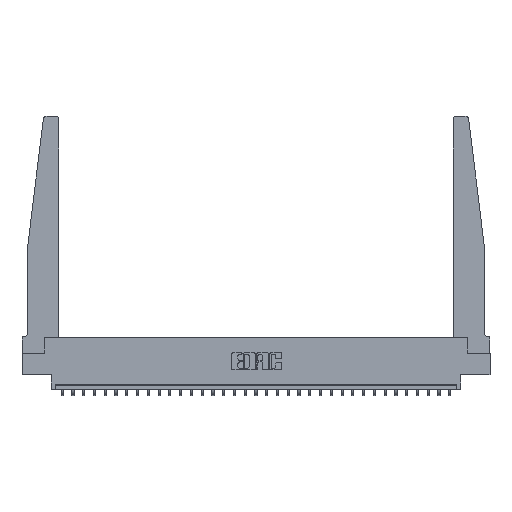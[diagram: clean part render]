
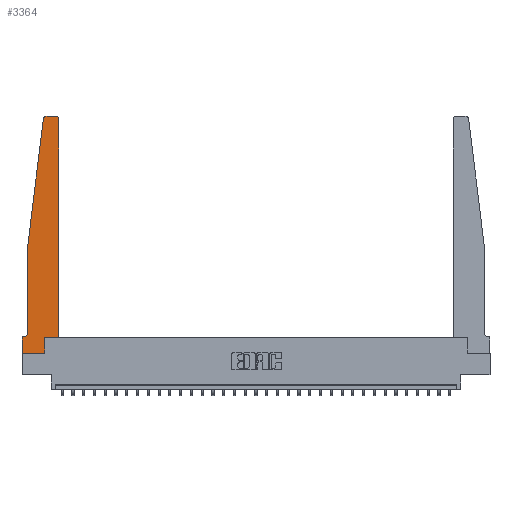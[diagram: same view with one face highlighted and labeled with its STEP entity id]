
A CAD part, top view. The second image highlights one B-rep face of the part: STEP entity #3364.
In plain terms, the highlighted planar face has unit normal (0, 0, 1).
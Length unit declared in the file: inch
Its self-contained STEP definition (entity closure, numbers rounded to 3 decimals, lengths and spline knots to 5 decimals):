
#192 = CARTESIAN_POINT ( 'NONE',  ( 0.24675, 2.72367, 0.37 ) ) ;
#817 = LINE ( 'NONE', #16457, #23224 ) ;
#862 = VECTOR ( 'NONE', #17582, 39.37008 ) ;
#1046 = CARTESIAN_POINT ( 'NONE',  ( 0.2605, 0.18, 0.37 ) ) ;
#1064 = PLANE ( 'NONE',  #9495 ) ;
#1229 = LINE ( 'NONE', #10339, #18105 ) ;
#1232 = ORIENTED_EDGE ( 'NONE', *, *, #4153, .T. ) ;
#2558 = ORIENTED_EDGE ( 'NONE', *, *, #18383, .T. ) ;
#2684 = VERTEX_POINT ( 'NONE', #6284 ) ;
#3140 = DIRECTION ( 'NONE',  ( 1., 0., 0. ) ) ;
#3364 = ADVANCED_FACE ( 'NONE', ( #12279 ), #1064, .T. ) ;
#4019 = DIRECTION ( 'NONE',  ( -1., 0., 0. ) ) ;
#4153 = EDGE_CURVE ( 'NONE', #28515, #22465, #817, .T. ) ;
#4591 = CARTESIAN_POINT ( 'NONE',  ( 0.27653, 2.75, 0.37 ) ) ;
#4769 = ORIENTED_EDGE ( 'NONE', *, *, #24922, .T. ) ;
#4983 = LINE ( 'NONE', #25038, #13120 ) ;
#5171 = VECTOR ( 'NONE', #12955, 39.37008 ) ;
#5205 = LINE ( 'NONE', #11398, #28593 ) ;
#5506 = CARTESIAN_POINT ( 'NONE',  ( 0.425, 0.18, 0.37 ) ) ;
#5631 = LINE ( 'NONE', #18643, #13634 ) ;
#5778 = EDGE_CURVE ( 'NONE', #22573, #10369, #5631, .T. ) ;
#5802 = CARTESIAN_POINT ( 'NONE',  ( 0., 0., 0.37 ) ) ;
#6070 = LINE ( 'NONE', #26667, #862 ) ;
#6284 = CARTESIAN_POINT ( 'NONE',  ( 0.395, 2.75, 0.37 ) ) ;
#6525 = DIRECTION ( 'NONE',  ( 0., 0., 1. ) ) ;
#6933 = EDGE_CURVE ( 'NONE', #2684, #7802, #19730, .T. ) ;
#7388 = CARTESIAN_POINT ( 'NONE',  ( 0., 0.1875, 0.37 ) ) ;
#7418 = AXIS2_PLACEMENT_3D ( 'NONE', #8844, #26550, #24643 ) ;
#7753 = ORIENTED_EDGE ( 'NONE', *, *, #6933, .T. ) ;
#7802 = VERTEX_POINT ( 'NONE', #4591 ) ;
#8844 = CARTESIAN_POINT ( 'NONE',  ( 0.27653, 2.72, 0.37 ) ) ;
#9439 = ORIENTED_EDGE ( 'NONE', *, *, #13994, .T. ) ;
#9495 = AXIS2_PLACEMENT_3D ( 'NONE', #7388, #27420, #16278 ) ;
#9849 = VERTEX_POINT ( 'NONE', #11634 ) ;
#9881 = ORIENTED_EDGE ( 'NONE', *, *, #18743, .T. ) ;
#9901 = ORIENTED_EDGE ( 'NONE', *, *, #19041, .T. ) ;
#10315 = EDGE_CURVE ( 'NONE', #22868, #20531, #14891, .T. ) ;
#10339 = CARTESIAN_POINT ( 'NONE',  ( 0.065, 0.1875, 0.37 ) ) ;
#10369 = VERTEX_POINT ( 'NONE', #24199 ) ;
#10718 = VERTEX_POINT ( 'NONE', #28671 ) ;
#10901 = ORIENTED_EDGE ( 'NONE', *, *, #13205, .T. ) ;
#11398 = CARTESIAN_POINT ( 'NONE',  ( 0., 0., 0.37 ) ) ;
#11634 = CARTESIAN_POINT ( 'NONE',  ( 0.425, 2.72, 0.37 ) ) ;
#12279 = FACE_OUTER_BOUND ( 'NONE', #26601, .T. ) ;
#12893 = DIRECTION ( 'NONE',  ( 1., 0., 0. ) ) ;
#12955 = DIRECTION ( 'NONE',  ( -1., 0., 0. ) ) ;
#13105 = CARTESIAN_POINT ( 'NONE',  ( 0.015, 0.1875, 0.37 ) ) ;
#13120 = VECTOR ( 'NONE', #22869, 39.37008 ) ;
#13168 = AXIS2_PLACEMENT_3D ( 'NONE', #24359, #6525, #12893 ) ;
#13205 = EDGE_CURVE ( 'NONE', #21389, #22868, #6070, .T. ) ;
#13335 = CARTESIAN_POINT ( 'NONE',  ( 0.065, 1.25, 0.37 ) ) ;
#13634 = VECTOR ( 'NONE', #3140, 39.37008 ) ;
#13673 = ORIENTED_EDGE ( 'NONE', *, *, #25592, .T. ) ;
#13994 = EDGE_CURVE ( 'NONE', #9849, #2684, #19753, .T. ) ;
#14057 = CIRCLE ( 'NONE', #7418, 0.03 ) ;
#14891 = CIRCLE ( 'NONE', #17257, 0.05 ) ;
#15223 = DIRECTION ( 'NONE',  ( -1., 0., 0. ) ) ;
#16278 = DIRECTION ( 'NONE',  ( 1., 0., 0. ) ) ;
#16457 = CARTESIAN_POINT ( 'NONE',  ( 0.425, 0.18, 0.37 ) ) ;
#16499 = DIRECTION ( 'NONE',  ( -0.122, -0.992, 0. ) ) ;
#17257 = AXIS2_PLACEMENT_3D ( 'NONE', #26807, #26518, #15223 ) ;
#17365 = VECTOR ( 'NONE', #19043, 39.37008 ) ;
#17582 = DIRECTION ( 'NONE',  ( 0., -1., 0. ) ) ;
#18105 = VECTOR ( 'NONE', #4019, 39.37008 ) ;
#18301 = VECTOR ( 'NONE', #16499, 39.37008 ) ;
#18383 = EDGE_CURVE ( 'NONE', #20531, #10718, #1229, .T. ) ;
#18413 = VERTEX_POINT ( 'NONE', #192 ) ;
#18419 = EDGE_CURVE ( 'NONE', #7802, #18413, #14057, .T. ) ;
#18643 = CARTESIAN_POINT ( 'NONE',  ( 0., 0., 0.37 ) ) ;
#18710 = LINE ( 'NONE', #21237, #18301 ) ;
#18743 = EDGE_CURVE ( 'NONE', #10369, #28515, #25925, .T. ) ;
#18768 = CARTESIAN_POINT ( 'NONE',  ( 0.065, 0.2375, 0.37 ) ) ;
#19041 = EDGE_CURVE ( 'NONE', #22465, #9849, #4983, .T. ) ;
#19043 = DIRECTION ( 'NONE',  ( 0., 1., 0. ) ) ;
#19730 = LINE ( 'NONE', #28351, #5171 ) ;
#19753 = CIRCLE ( 'NONE', #13168, 0.03 ) ;
#20531 = VERTEX_POINT ( 'NONE', #13105 ) ;
#21237 = CARTESIAN_POINT ( 'NONE',  ( 0.065, 1.25, 0.37 ) ) ;
#21389 = VERTEX_POINT ( 'NONE', #13335 ) ;
#21995 = ORIENTED_EDGE ( 'NONE', *, *, #18419, .T. ) ;
#22465 = VERTEX_POINT ( 'NONE', #5506 ) ;
#22521 = ORIENTED_EDGE ( 'NONE', *, *, #10315, .T. ) ;
#22573 = VERTEX_POINT ( 'NONE', #5802 ) ;
#22868 = VERTEX_POINT ( 'NONE', #18768 ) ;
#22869 = DIRECTION ( 'NONE',  ( 0., 1., 0. ) ) ;
#22904 = CARTESIAN_POINT ( 'NONE',  ( 0.2605, 0.18, 0.37 ) ) ;
#23216 = DIRECTION ( 'NONE',  ( 0., -1., 0. ) ) ;
#23224 = VECTOR ( 'NONE', #25692, 39.37008 ) ;
#24199 = CARTESIAN_POINT ( 'NONE',  ( 0.2605, 0., 0.37 ) ) ;
#24359 = CARTESIAN_POINT ( 'NONE',  ( 0.395, 2.72, 0.37 ) ) ;
#24643 = DIRECTION ( 'NONE',  ( 1., 0., 0. ) ) ;
#24922 = EDGE_CURVE ( 'NONE', #18413, #21389, #18710, .T. ) ;
#25038 = CARTESIAN_POINT ( 'NONE',  ( 0.425, 0.18, 0.37 ) ) ;
#25592 = EDGE_CURVE ( 'NONE', #10718, #22573, #5205, .T. ) ;
#25692 = DIRECTION ( 'NONE',  ( 1., 0., 0. ) ) ;
#25784 = ORIENTED_EDGE ( 'NONE', *, *, #5778, .T. ) ;
#25925 = LINE ( 'NONE', #1046, #17365 ) ;
#26518 = DIRECTION ( 'NONE',  ( 0., 0., -1. ) ) ;
#26550 = DIRECTION ( 'NONE',  ( 0., 0., 1. ) ) ;
#26601 = EDGE_LOOP ( 'NONE', ( #7753, #21995, #4769, #10901, #22521, #2558, #13673, #25784, #9881, #1232, #9901, #9439 ) ) ;
#26667 = CARTESIAN_POINT ( 'NONE',  ( 0.065, 1.25, 0.37 ) ) ;
#26807 = CARTESIAN_POINT ( 'NONE',  ( 0.015, 0.2375, 0.37 ) ) ;
#27420 = DIRECTION ( 'NONE',  ( 0., 0., 1. ) ) ;
#28351 = CARTESIAN_POINT ( 'NONE',  ( 0.25, 2.75, 0.37 ) ) ;
#28515 = VERTEX_POINT ( 'NONE', #22904 ) ;
#28593 = VECTOR ( 'NONE', #23216, 39.37008 ) ;
#28671 = CARTESIAN_POINT ( 'NONE',  ( 0., 0.1875, 0.37 ) ) ;
